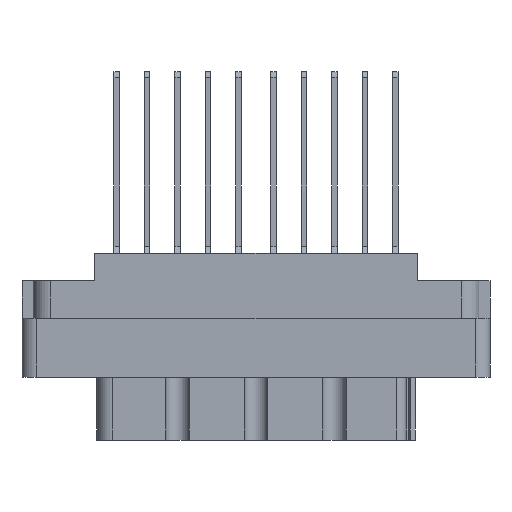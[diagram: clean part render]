
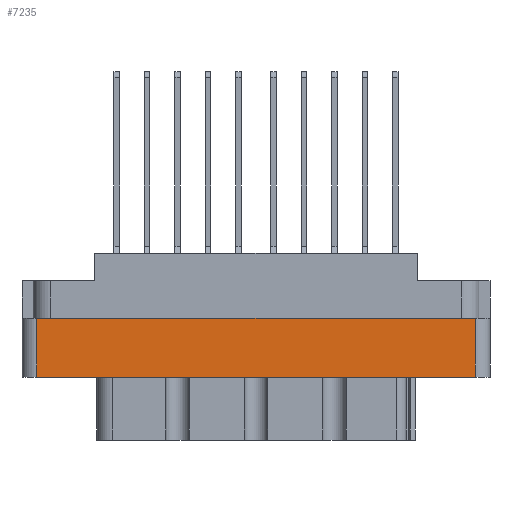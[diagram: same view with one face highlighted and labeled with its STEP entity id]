
A CAD part, front view. The second image highlights one B-rep face of the part: STEP entity #7235.
In plain terms, the highlighted planar face has unit normal (0, -1, 0).
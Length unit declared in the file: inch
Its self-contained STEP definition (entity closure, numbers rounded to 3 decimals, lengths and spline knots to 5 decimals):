
#205 = LINE ( 'NONE', #21160, #10282 ) ;
#2144 = DIRECTION ( 'NONE',  ( 1., 0., 0. ) ) ;
#2305 = DIRECTION ( 'NONE',  ( 0., 0., 1. ) ) ;
#2407 = CARTESIAN_POINT ( 'NONE',  ( -0.938, -0.438, -0.798 ) ) ;
#4087 = LINE ( 'NONE', #29183, #26654 ) ;
#6020 = CARTESIAN_POINT ( 'NONE',  ( -1., -0.438, -0.798 ) ) ;
#7235 = ADVANCED_FACE ( 'NONE', ( #10489 ), #19248, .T. ) ;
#7799 = LINE ( 'NONE', #33069, #11554 ) ;
#8029 = CARTESIAN_POINT ( 'NONE',  ( -0.938, -0.438, -0.529 ) ) ;
#8202 = AXIS2_PLACEMENT_3D ( 'NONE', #6020, #32637, #27183 ) ;
#8403 = EDGE_LOOP ( 'NONE', ( #10895, #17758, #8602, #26186 ) ) ;
#8602 = ORIENTED_EDGE ( 'NONE', *, *, #10025, .F. ) ;
#8672 = EDGE_CURVE ( 'NONE', #28611, #30903, #32671, .T. ) ;
#10025 = EDGE_CURVE ( 'NONE', #29224, #30903, #7799, .T. ) ;
#10282 = VECTOR ( 'NONE', #2305, 39.37008 ) ;
#10489 = FACE_OUTER_BOUND ( 'NONE', #8403, .T. ) ;
#10895 = ORIENTED_EDGE ( 'NONE', *, *, #24315, .F. ) ;
#11554 = VECTOR ( 'NONE', #14641, 39.37008 ) ;
#12571 = CARTESIAN_POINT ( 'NONE',  ( 0.938, -0.438, -0.277 ) ) ;
#14641 = DIRECTION ( 'NONE',  ( -1., 0., 0. ) ) ;
#16178 = CARTESIAN_POINT ( 'NONE',  ( 0.938, -0.438, -0.529 ) ) ;
#16949 = EDGE_CURVE ( 'NONE', #29224, #18280, #205, .T. ) ;
#17758 = ORIENTED_EDGE ( 'NONE', *, *, #8672, .T. ) ;
#18280 = VERTEX_POINT ( 'NONE', #12571 ) ;
#19248 = PLANE ( 'NONE',  #8202 ) ;
#21160 = CARTESIAN_POINT ( 'NONE',  ( 0.938, -0.438, -0.798 ) ) ;
#23835 = DIRECTION ( 'NONE',  ( 0., 0., -1. ) ) ;
#24315 = EDGE_CURVE ( 'NONE', #28611, #18280, #4087, .T. ) ;
#26186 = ORIENTED_EDGE ( 'NONE', *, *, #16949, .T. ) ;
#26333 = VECTOR ( 'NONE', #23835, 39.37008 ) ;
#26654 = VECTOR ( 'NONE', #2144, 39.37008 ) ;
#27183 = DIRECTION ( 'NONE',  ( 0., 0., -1. ) ) ;
#27208 = CARTESIAN_POINT ( 'NONE',  ( -0.938, -0.438, -0.277 ) ) ;
#28611 = VERTEX_POINT ( 'NONE', #27208 ) ;
#29183 = CARTESIAN_POINT ( 'NONE',  ( 0., -0.438, -0.277 ) ) ;
#29224 = VERTEX_POINT ( 'NONE', #16178 ) ;
#30903 = VERTEX_POINT ( 'NONE', #8029 ) ;
#32637 = DIRECTION ( 'NONE',  ( 0., -1., 0. ) ) ;
#32671 = LINE ( 'NONE', #2407, #26333 ) ;
#33069 = CARTESIAN_POINT ( 'NONE',  ( 0., -0.438, -0.529 ) ) ;
